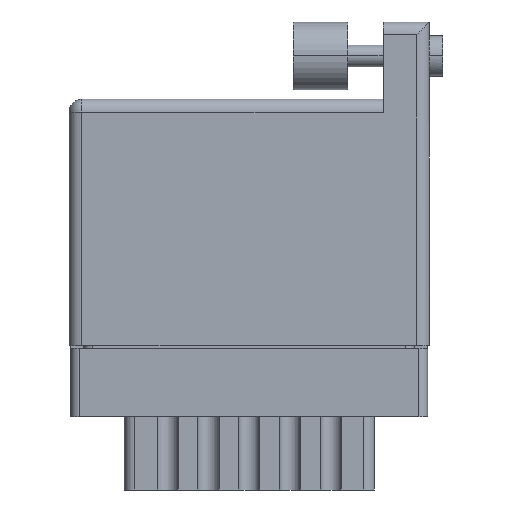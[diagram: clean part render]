
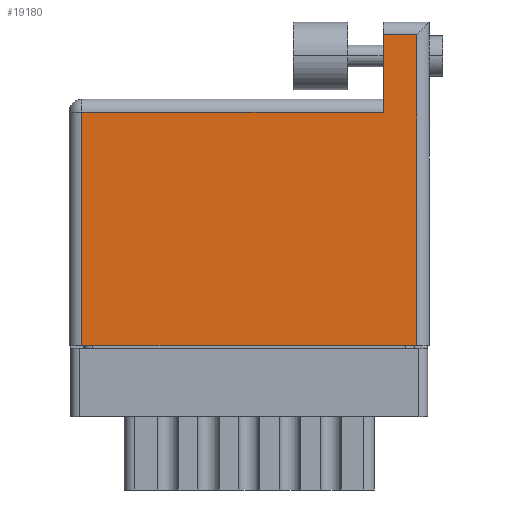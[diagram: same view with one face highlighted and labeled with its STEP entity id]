
A CAD part, front view. The second image highlights one B-rep face of the part: STEP entity #19180.
In plain terms, the highlighted face is planar.
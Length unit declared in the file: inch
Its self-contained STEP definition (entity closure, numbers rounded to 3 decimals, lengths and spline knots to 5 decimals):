
#312 = DIRECTION ( 'NONE',  ( 0., -1., 0. ) ) ;
#320 = EDGE_CURVE ( 'NONE', #17893, #12063, #24004, .T. ) ;
#739 = CARTESIAN_POINT ( 'NONE',  ( 1.155, 1.143, 0. ) ) ;
#1166 = ORIENTED_EDGE ( 'NONE', *, *, #22010, .T. ) ;
#1930 = EDGE_CURVE ( 'NONE', #12063, #23627, #12225, .T. ) ;
#3682 = CARTESIAN_POINT ( 'NONE',  ( 1.278, 1.19, 0. ) ) ;
#3767 = EDGE_LOOP ( 'NONE', ( #14103, #22083, #5147, #9897, #1166, #13480 ) ) ;
#4462 = CARTESIAN_POINT ( 'NONE',  ( 0., 0.906, 0. ) ) ;
#5147 = ORIENTED_EDGE ( 'NONE', *, *, #320, .T. ) ;
#5266 = DIRECTION ( 'NONE',  ( -1., 0., 0. ) ) ;
#6114 = VERTEX_POINT ( 'NONE', #10389 ) ;
#6415 = EDGE_CURVE ( 'NONE', #17978, #17893, #23977, .T. ) ;
#6573 = VECTOR ( 'NONE', #312, 39.37008 ) ;
#9897 = ORIENTED_EDGE ( 'NONE', *, *, #1930, .T. ) ;
#10389 = CARTESIAN_POINT ( 'NONE',  ( 0.047, 0.859, 0. ) ) ;
#10944 = VERTEX_POINT ( 'NONE', #17380 ) ;
#11109 = CARTESIAN_POINT ( 'NONE',  ( 1.155, 1.143, 0. ) ) ;
#11568 = DIRECTION ( 'NONE',  ( 0., 1., 0. ) ) ;
#12063 = VERTEX_POINT ( 'NONE', #739 ) ;
#12225 = LINE ( 'NONE', #18453, #6573 ) ;
#12422 = DIRECTION ( 'NONE',  ( 0., -1., 0. ) ) ;
#12478 = CARTESIAN_POINT ( 'NONE',  ( 1.278, 0., 0. ) ) ;
#12586 = PLANE ( 'NONE',  #17207 ) ;
#13480 = ORIENTED_EDGE ( 'NONE', *, *, #23084, .T. ) ;
#13603 = VECTOR ( 'NONE', #5266, 39.37008 ) ;
#13877 = VECTOR ( 'NONE', #11568, 39.37008 ) ;
#14103 = ORIENTED_EDGE ( 'NONE', *, *, #21980, .T. ) ;
#14648 = LINE ( 'NONE', #19241, #20921 ) ;
#15282 = CARTESIAN_POINT ( 'NONE',  ( 0., 0.859, 0. ) ) ;
#15542 = LINE ( 'NONE', #15282, #22832 ) ;
#16576 = DIRECTION ( 'NONE',  ( -1., 0., 0. ) ) ;
#17207 = AXIS2_PLACEMENT_3D ( 'NONE', #4462, #22384, #16576 ) ;
#17251 = DIRECTION ( 'NONE',  ( 1., 0., 0. ) ) ;
#17380 = CARTESIAN_POINT ( 'NONE',  ( 0.047, 0., 0. ) ) ;
#17893 = VERTEX_POINT ( 'NONE', #22954 ) ;
#17978 = VERTEX_POINT ( 'NONE', #12478 ) ;
#18453 = CARTESIAN_POINT ( 'NONE',  ( 1.155, 1.19, 0. ) ) ;
#19180 = ADVANCED_FACE ( 'NONE', ( #21196 ), #12586, .F. ) ;
#19241 = CARTESIAN_POINT ( 'NONE',  ( 0., 0., 0. ) ) ;
#20198 = VECTOR ( 'NONE', #12422, 39.37008 ) ;
#20840 = LINE ( 'NONE', #24506, #20198 ) ;
#20921 = VECTOR ( 'NONE', #17251, 39.37008 ) ;
#21196 = FACE_OUTER_BOUND ( 'NONE', #3767, .T. ) ;
#21980 = EDGE_CURVE ( 'NONE', #10944, #17978, #14648, .T. ) ;
#22010 = EDGE_CURVE ( 'NONE', #23627, #6114, #15542, .T. ) ;
#22083 = ORIENTED_EDGE ( 'NONE', *, *, #6415, .T. ) ;
#22384 = DIRECTION ( 'NONE',  ( 0., 0., -1. ) ) ;
#22626 = CARTESIAN_POINT ( 'NONE',  ( 1.155, 0.859, 0. ) ) ;
#22832 = VECTOR ( 'NONE', #23142, 39.37008 ) ;
#22954 = CARTESIAN_POINT ( 'NONE',  ( 1.278, 1.143, 0. ) ) ;
#23084 = EDGE_CURVE ( 'NONE', #6114, #10944, #20840, .T. ) ;
#23142 = DIRECTION ( 'NONE',  ( -1., 0., 0. ) ) ;
#23627 = VERTEX_POINT ( 'NONE', #22626 ) ;
#23977 = LINE ( 'NONE', #3682, #13877 ) ;
#24004 = LINE ( 'NONE', #11109, #13603 ) ;
#24506 = CARTESIAN_POINT ( 'NONE',  ( 0.047, 0., 0. ) ) ;
